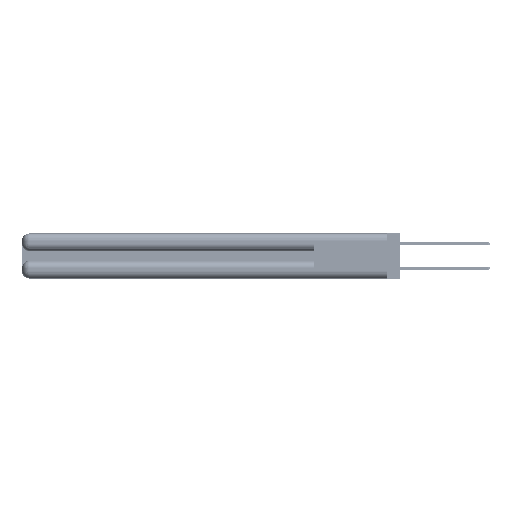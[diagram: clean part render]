
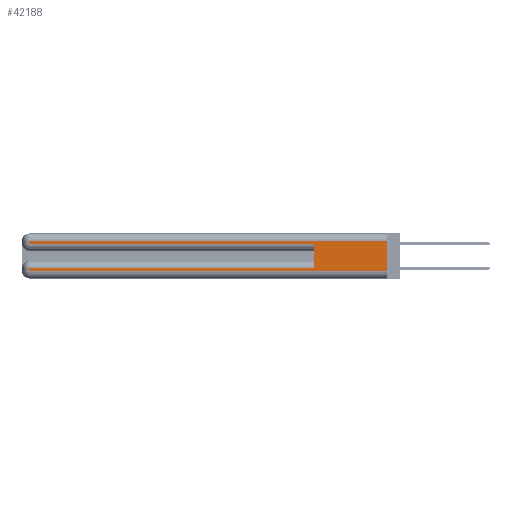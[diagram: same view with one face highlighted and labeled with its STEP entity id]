
A CAD part, left-side view. The second image highlights one B-rep face of the part: STEP entity #42188.
In plain terms, the highlighted planar face has unit normal (-1, 0, 0).
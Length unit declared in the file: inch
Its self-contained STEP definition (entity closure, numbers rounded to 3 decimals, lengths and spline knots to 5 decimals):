
#479 = VECTOR ( 'NONE', #46271, 39.37008 ) ;
#1149 = LINE ( 'NONE', #42590, #479 ) ;
#3265 = CARTESIAN_POINT ( 'NONE',  ( 0., 0., 0.31 ) ) ;
#4185 = VECTOR ( 'NONE', #13797, 39.37008 ) ;
#4587 = CARTESIAN_POINT ( 'NONE',  ( 0., 0., 0.085 ) ) ;
#5022 = ORIENTED_EDGE ( 'NONE', *, *, #56284, .F. ) ;
#5594 = CARTESIAN_POINT ( 'NONE',  ( 0., 0.6, 0.085 ) ) ;
#5706 = ORIENTED_EDGE ( 'NONE', *, *, #47884, .T. ) ;
#5982 = PLANE ( 'NONE',  #25703 ) ;
#8015 = VECTOR ( 'NONE', #9012, 39.37008 ) ;
#9012 = DIRECTION ( 'NONE',  ( 0., -1., 0. ) ) ;
#9895 = VERTEX_POINT ( 'NONE', #14019 ) ;
#10978 = CARTESIAN_POINT ( 'NONE',  ( 0., 0.6, 0.285 ) ) ;
#12448 = VERTEX_POINT ( 'NONE', #5594 ) ;
#12502 = VECTOR ( 'NONE', #16683, 39.37008 ) ;
#13147 = EDGE_LOOP ( 'NONE', ( #36809, #24639, #14001, #53235, #5022, #15258, #5706, #21522 ) ) ;
#13231 = VERTEX_POINT ( 'NONE', #39340 ) ;
#13797 = DIRECTION ( 'NONE',  ( 0., 1., 0. ) ) ;
#14001 = ORIENTED_EDGE ( 'NONE', *, *, #14349, .T. ) ;
#14019 = CARTESIAN_POINT ( 'NONE',  ( 0., 2.94, 0.06 ) ) ;
#14149 = VERTEX_POINT ( 'NONE', #10978 ) ;
#14349 = EDGE_CURVE ( 'NONE', #47749, #36503, #51374, .T. ) ;
#15164 = DIRECTION ( 'NONE',  ( 0., 0., 1. ) ) ;
#15258 = ORIENTED_EDGE ( 'NONE', *, *, #30026, .T. ) ;
#16683 = DIRECTION ( 'NONE',  ( 0., 1., 0. ) ) ;
#19655 = LINE ( 'NONE', #22042, #8015 ) ;
#21063 = VECTOR ( 'NONE', #15164, 39.37008 ) ;
#21522 = ORIENTED_EDGE ( 'NONE', *, *, #56693, .T. ) ;
#22042 = CARTESIAN_POINT ( 'NONE',  ( 0., 0., 0.06 ) ) ;
#23170 = LINE ( 'NONE', #47410, #44473 ) ;
#23369 = EDGE_CURVE ( 'NONE', #50147, #45873, #1149, .T. ) ;
#23510 = CARTESIAN_POINT ( 'NONE',  ( 0., 0., 0.31 ) ) ;
#24639 = ORIENTED_EDGE ( 'NONE', *, *, #51368, .T. ) ;
#25703 = AXIS2_PLACEMENT_3D ( 'NONE', #49819, #45571, #54202 ) ;
#26053 = EDGE_CURVE ( 'NONE', #36503, #14149, #47629, .T. ) ;
#26868 = CARTESIAN_POINT ( 'NONE',  ( 0., 0., 0.06 ) ) ;
#28371 = VECTOR ( 'NONE', #33997, 39.37008 ) ;
#30026 = EDGE_CURVE ( 'NONE', #12448, #13231, #32388, .T. ) ;
#30288 = DIRECTION ( 'NONE',  ( 0., 0., -1. ) ) ;
#32319 = CARTESIAN_POINT ( 'NONE',  ( 0., 0.6, 0.145 ) ) ;
#32388 = LINE ( 'NONE', #4587, #4185 ) ;
#32821 = LINE ( 'NONE', #32319, #21063 ) ;
#33526 = VECTOR ( 'NONE', #51149, 39.37008 ) ;
#33997 = DIRECTION ( 'NONE',  ( 0., -1., 0. ) ) ;
#34183 = CARTESIAN_POINT ( 'NONE',  ( 0., 0., 0.285 ) ) ;
#36503 = VERTEX_POINT ( 'NONE', #44588 ) ;
#36809 = ORIENTED_EDGE ( 'NONE', *, *, #23369, .F. ) ;
#37894 = CARTESIAN_POINT ( 'NONE',  ( 0., 2.94, 0.37 ) ) ;
#39340 = CARTESIAN_POINT ( 'NONE',  ( 0., 2.94, 0.085 ) ) ;
#42188 = ADVANCED_FACE ( 'NONE', ( #49802 ), #5982, .F. ) ;
#42213 = CARTESIAN_POINT ( 'NONE',  ( 0., 2.94, 0.31 ) ) ;
#42590 = CARTESIAN_POINT ( 'NONE',  ( 0., 0., 0.37 ) ) ;
#44473 = VECTOR ( 'NONE', #30288, 39.37008 ) ;
#44588 = CARTESIAN_POINT ( 'NONE',  ( 0., 2.94, 0.285 ) ) ;
#45500 = LINE ( 'NONE', #3265, #12502 ) ;
#45571 = DIRECTION ( 'NONE',  ( 1., 0., 0. ) ) ;
#45873 = VERTEX_POINT ( 'NONE', #26868 ) ;
#46271 = DIRECTION ( 'NONE',  ( 0., 0., -1. ) ) ;
#47410 = CARTESIAN_POINT ( 'NONE',  ( 0., 2.94, 0.37 ) ) ;
#47629 = LINE ( 'NONE', #34183, #28371 ) ;
#47749 = VERTEX_POINT ( 'NONE', #42213 ) ;
#47884 = EDGE_CURVE ( 'NONE', #13231, #9895, #23170, .T. ) ;
#49802 = FACE_OUTER_BOUND ( 'NONE', #13147, .T. ) ;
#49819 = CARTESIAN_POINT ( 'NONE',  ( 0., 0., 0.37 ) ) ;
#50147 = VERTEX_POINT ( 'NONE', #23510 ) ;
#51149 = DIRECTION ( 'NONE',  ( 0., 0., -1. ) ) ;
#51368 = EDGE_CURVE ( 'NONE', #50147, #47749, #45500, .T. ) ;
#51374 = LINE ( 'NONE', #37894, #33526 ) ;
#53235 = ORIENTED_EDGE ( 'NONE', *, *, #26053, .T. ) ;
#54202 = DIRECTION ( 'NONE',  ( 0., 0., -1. ) ) ;
#56284 = EDGE_CURVE ( 'NONE', #12448, #14149, #32821, .T. ) ;
#56693 = EDGE_CURVE ( 'NONE', #9895, #45873, #19655, .T. ) ;
